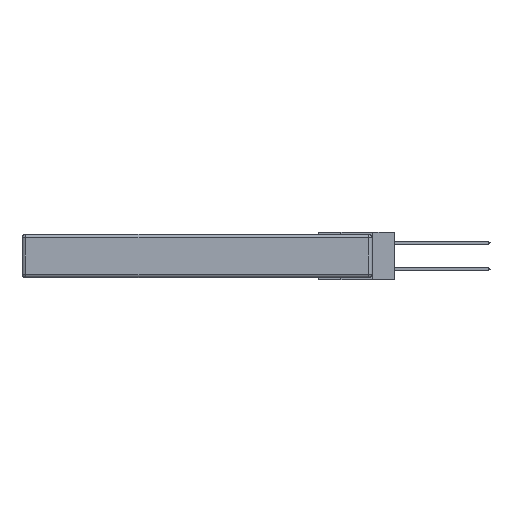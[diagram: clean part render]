
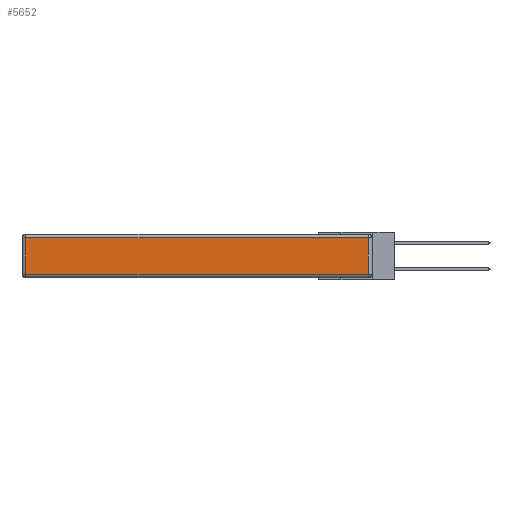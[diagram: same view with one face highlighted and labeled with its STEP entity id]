
A CAD part, left-side view. The second image highlights one B-rep face of the part: STEP entity #5652.
In plain terms, the highlighted planar face has unit normal (-1, 0, 0).
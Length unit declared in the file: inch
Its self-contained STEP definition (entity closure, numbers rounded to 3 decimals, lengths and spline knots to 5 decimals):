
#1033 = FACE_OUTER_BOUND ( 'NONE', #5850, .T. ) ;
#2063 = VERTEX_POINT ( 'NONE', #33939 ) ;
#2079 = DIRECTION ( 'NONE',  ( 0., 0., 1. ) ) ;
#2383 = LINE ( 'NONE', #25486, #18709 ) ;
#4069 = DIRECTION ( 'NONE',  ( 0., -1., 0. ) ) ;
#4579 = VERTEX_POINT ( 'NONE', #28113 ) ;
#5652 = ADVANCED_FACE ( 'NONE', ( #1033 ), #25291, .T. ) ;
#5850 = EDGE_LOOP ( 'NONE', ( #10051, #14592, #14251, #21311 ) ) ;
#5877 = EDGE_CURVE ( 'NONE', #4579, #2063, #21903, .T. ) ;
#7571 = CARTESIAN_POINT ( 'NONE',  ( 0., 2.72, -0.343 ) ) ;
#8422 = CARTESIAN_POINT ( 'NONE',  ( 0., 0.03, -0.03 ) ) ;
#9043 = LINE ( 'NONE', #19463, #28349 ) ;
#10051 = ORIENTED_EDGE ( 'NONE', *, *, #14716, .T. ) ;
#10404 = DIRECTION ( 'NONE',  ( 0., 0., -1. ) ) ;
#11378 = EDGE_CURVE ( 'NONE', #17081, #4579, #9043, .T. ) ;
#14251 = ORIENTED_EDGE ( 'NONE', *, *, #11378, .T. ) ;
#14592 = ORIENTED_EDGE ( 'NONE', *, *, #17330, .T. ) ;
#14716 = EDGE_CURVE ( 'NONE', #2063, #16556, #2383, .T. ) ;
#16524 = DIRECTION ( 'NONE',  ( 0., 1., 0. ) ) ;
#16556 = VERTEX_POINT ( 'NONE', #28010 ) ;
#17081 = VERTEX_POINT ( 'NONE', #8422 ) ;
#17330 = EDGE_CURVE ( 'NONE', #16556, #17081, #23423, .T. ) ;
#17466 = DIRECTION ( 'NONE',  ( 0., 0., 1. ) ) ;
#18709 = VECTOR ( 'NONE', #4069, 39.37008 ) ;
#19463 = CARTESIAN_POINT ( 'NONE',  ( 0., 2.75, -0.03 ) ) ;
#21311 = ORIENTED_EDGE ( 'NONE', *, *, #5877, .T. ) ;
#21903 = LINE ( 'NONE', #7571, #33208 ) ;
#22833 = DIRECTION ( 'NONE',  ( -1., 0., 0. ) ) ;
#23271 = CARTESIAN_POINT ( 'NONE',  ( 0., 0.03, -0.343 ) ) ;
#23423 = LINE ( 'NONE', #23271, #29318 ) ;
#25291 = PLANE ( 'NONE',  #33389 ) ;
#25486 = CARTESIAN_POINT ( 'NONE',  ( 0., 0., -0.313 ) ) ;
#25851 = CARTESIAN_POINT ( 'NONE',  ( 0., 0., -0.343 ) ) ;
#28010 = CARTESIAN_POINT ( 'NONE',  ( 0., 0.03, -0.313 ) ) ;
#28113 = CARTESIAN_POINT ( 'NONE',  ( 0., 2.72, -0.03 ) ) ;
#28349 = VECTOR ( 'NONE', #16524, 39.37008 ) ;
#29318 = VECTOR ( 'NONE', #2079, 39.37008 ) ;
#33208 = VECTOR ( 'NONE', #10404, 39.37008 ) ;
#33389 = AXIS2_PLACEMENT_3D ( 'NONE', #25851, #22833, #17466 ) ;
#33939 = CARTESIAN_POINT ( 'NONE',  ( 0., 2.72, -0.313 ) ) ;
